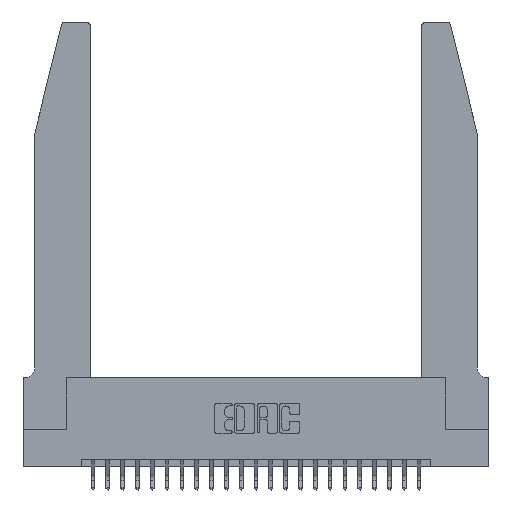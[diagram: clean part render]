
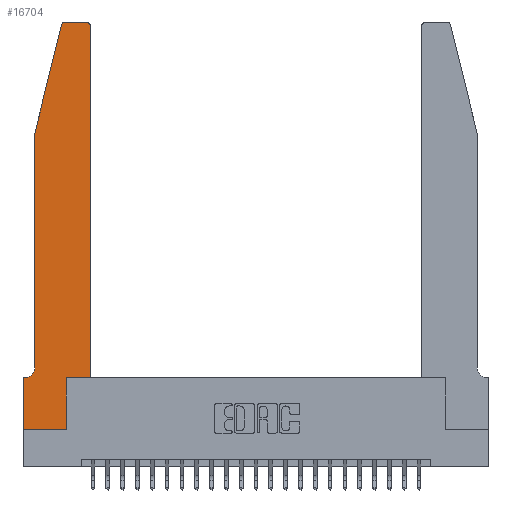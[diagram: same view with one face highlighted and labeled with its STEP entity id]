
A CAD part, top view. The second image highlights one B-rep face of the part: STEP entity #16704.
In plain terms, the highlighted planar face has unit normal (0, 0, 1).
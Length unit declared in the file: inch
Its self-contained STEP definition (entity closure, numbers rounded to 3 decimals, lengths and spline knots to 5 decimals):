
#554 = VERTEX_POINT ( 'NONE', #5459 ) ;
#1057 = EDGE_CURVE ( 'NONE', #1866, #18185, #18213, .T. ) ;
#1120 = ORIENTED_EDGE ( 'NONE', *, *, #1057, .T. ) ;
#1135 = DIRECTION ( 'NONE',  ( 0., 1., 0. ) ) ;
#1212 = DIRECTION ( 'NONE',  ( 0., 0., 1. ) ) ;
#1472 = VECTOR ( 'NONE', #25220, 39.37008 ) ;
#1668 = ORIENTED_EDGE ( 'NONE', *, *, #20051, .T. ) ;
#1866 = VERTEX_POINT ( 'NONE', #25402 ) ;
#1999 = EDGE_LOOP ( 'NONE', ( #12374, #14476, #10716, #1668, #5855, #5025, #1120, #21584, #4840, #23138, #11516, #9669 ) ) ;
#2002 = VECTOR ( 'NONE', #21650, 39.37008 ) ;
#2363 = VECTOR ( 'NONE', #12882, 39.37008 ) ;
#2982 = CARTESIAN_POINT ( 'NONE',  ( 0.4505, 0.35, 0.37 ) ) ;
#3027 = FACE_OUTER_BOUND ( 'NONE', #1999, .T. ) ;
#3102 = CARTESIAN_POINT ( 'NONE',  ( 0.2865, 0.35, 0.37 ) ) ;
#3235 = EDGE_CURVE ( 'NONE', #9959, #17209, #5210, .T. ) ;
#3626 = VECTOR ( 'NONE', #8977, 39.37008 ) ;
#4142 = VECTOR ( 'NONE', #10267, 39.37008 ) ;
#4840 = ORIENTED_EDGE ( 'NONE', *, *, #15202, .T. ) ;
#5025 = ORIENTED_EDGE ( 'NONE', *, *, #18685, .T. ) ;
#5210 = LINE ( 'NONE', #7529, #14553 ) ;
#5345 = EDGE_CURVE ( 'NONE', #22620, #9959, #12611, .T. ) ;
#5459 = CARTESIAN_POINT ( 'NONE',  ( 0.2865, 0., 0.37 ) ) ;
#5855 = ORIENTED_EDGE ( 'NONE', *, *, #17595, .T. ) ;
#5889 = CIRCLE ( 'NONE', #6001, 0.07 ) ;
#6001 = AXIS2_PLACEMENT_3D ( 'NONE', #19806, #8163, #21747 ) ;
#6195 = VECTOR ( 'NONE', #22273, 39.37008 ) ;
#6273 = CARTESIAN_POINT ( 'NONE',  ( 0.4205, 2.72, 0.37 ) ) ;
#6598 = CARTESIAN_POINT ( 'NONE',  ( 0.25487, 2.72718, 0.37 ) ) ;
#7315 = VERTEX_POINT ( 'NONE', #19235 ) ;
#7410 = VERTEX_POINT ( 'NONE', #11855 ) ;
#7475 = LINE ( 'NONE', #10089, #2002 ) ;
#7529 = CARTESIAN_POINT ( 'NONE',  ( 0.4505, 0.35, 0.37 ) ) ;
#7769 = CARTESIAN_POINT ( 'NONE',  ( 0.0755, 0.35, 0.37 ) ) ;
#8083 = CIRCLE ( 'NONE', #14499, 0.03 ) ;
#8146 = CARTESIAN_POINT ( 'NONE',  ( 0., 0., 0.37 ) ) ;
#8163 = DIRECTION ( 'NONE',  ( 0., 0., -1. ) ) ;
#8234 = CIRCLE ( 'NONE', #23222, 0.03 ) ;
#8270 = DIRECTION ( 'NONE',  ( 1., 0., 0. ) ) ;
#8977 = DIRECTION ( 'NONE',  ( 1., 0., 0. ) ) ;
#9244 = EDGE_CURVE ( 'NONE', #18185, #554, #14301, .T. ) ;
#9580 = CARTESIAN_POINT ( 'NONE',  ( 0.284, 2.72, 0.37 ) ) ;
#9669 = ORIENTED_EDGE ( 'NONE', *, *, #24172, .T. ) ;
#9959 = VERTEX_POINT ( 'NONE', #2982 ) ;
#10089 = CARTESIAN_POINT ( 'NONE',  ( 0.0755, 2., 0.37 ) ) ;
#10267 = DIRECTION ( 'NONE',  ( -0.239, -0.971, 0. ) ) ;
#10716 = ORIENTED_EDGE ( 'NONE', *, *, #11578, .T. ) ;
#11509 = LINE ( 'NONE', #16530, #6195 ) ;
#11516 = ORIENTED_EDGE ( 'NONE', *, *, #3235, .T. ) ;
#11578 = EDGE_CURVE ( 'NONE', #16018, #12915, #14186, .T. ) ;
#11592 = DIRECTION ( 'NONE',  ( 1., 0., 0. ) ) ;
#11786 = CARTESIAN_POINT ( 'NONE',  ( 0.2865, 0.35, 0.37 ) ) ;
#11855 = CARTESIAN_POINT ( 'NONE',  ( 0.0055, 0.35, 0.37 ) ) ;
#12374 = ORIENTED_EDGE ( 'NONE', *, *, #17781, .T. ) ;
#12384 = CARTESIAN_POINT ( 'NONE',  ( 0.284, 2.75, 0.37 ) ) ;
#12611 = LINE ( 'NONE', #13923, #17730 ) ;
#12840 = AXIS2_PLACEMENT_3D ( 'NONE', #20936, #1212, #15321 ) ;
#12882 = DIRECTION ( 'NONE',  ( 0., -1., 0. ) ) ;
#12915 = VERTEX_POINT ( 'NONE', #17141 ) ;
#13000 = CARTESIAN_POINT ( 'NONE',  ( 0.4505, 2.72, 0.37 ) ) ;
#13360 = PLANE ( 'NONE',  #12840 ) ;
#13923 = CARTESIAN_POINT ( 'NONE',  ( 0.4505, 0.35, 0.37 ) ) ;
#14101 = VECTOR ( 'NONE', #19444, 39.37008 ) ;
#14148 = CARTESIAN_POINT ( 'NONE',  ( 0., 0., 0.37 ) ) ;
#14186 = LINE ( 'NONE', #21837, #4142 ) ;
#14301 = LINE ( 'NONE', #16787, #3626 ) ;
#14476 = ORIENTED_EDGE ( 'NONE', *, *, #17411, .T. ) ;
#14499 = AXIS2_PLACEMENT_3D ( 'NONE', #9580, #23107, #11592 ) ;
#14553 = VECTOR ( 'NONE', #1135, 39.37008 ) ;
#15202 = EDGE_CURVE ( 'NONE', #554, #22620, #21880, .T. ) ;
#15321 = DIRECTION ( 'NONE',  ( 1., 0., 0. ) ) ;
#16018 = VERTEX_POINT ( 'NONE', #6598 ) ;
#16530 = CARTESIAN_POINT ( 'NONE',  ( 0.2605, 2.75, 0.37 ) ) ;
#16704 = ADVANCED_FACE ( 'NONE', ( #3027 ), #13360, .T. ) ;
#16787 = CARTESIAN_POINT ( 'NONE',  ( 0., 0., 0.37 ) ) ;
#17141 = CARTESIAN_POINT ( 'NONE',  ( 0.0755, 2., 0.37 ) ) ;
#17209 = VERTEX_POINT ( 'NONE', #13000 ) ;
#17411 = EDGE_CURVE ( 'NONE', #20614, #16018, #8083, .T. ) ;
#17595 = EDGE_CURVE ( 'NONE', #7315, #7410, #5889, .T. ) ;
#17730 = VECTOR ( 'NONE', #19635, 39.37008 ) ;
#17781 = EDGE_CURVE ( 'NONE', #23366, #20614, #11509, .T. ) ;
#18185 = VERTEX_POINT ( 'NONE', #8146 ) ;
#18213 = LINE ( 'NONE', #14148, #2363 ) ;
#18552 = LINE ( 'NONE', #7769, #14101 ) ;
#18685 = EDGE_CURVE ( 'NONE', #7410, #1866, #18552, .T. ) ;
#19235 = CARTESIAN_POINT ( 'NONE',  ( 0.0755, 0.42, 0.37 ) ) ;
#19444 = DIRECTION ( 'NONE',  ( -1., 0., 0. ) ) ;
#19635 = DIRECTION ( 'NONE',  ( 1., 0., 0. ) ) ;
#19806 = CARTESIAN_POINT ( 'NONE',  ( 0.0055, 0.42, 0.37 ) ) ;
#19895 = DIRECTION ( 'NONE',  ( 0., 0., 1. ) ) ;
#20051 = EDGE_CURVE ( 'NONE', #12915, #7315, #7475, .T. ) ;
#20614 = VERTEX_POINT ( 'NONE', #12384 ) ;
#20936 = CARTESIAN_POINT ( 'NONE',  ( 0., 0.35, 0.37 ) ) ;
#21584 = ORIENTED_EDGE ( 'NONE', *, *, #9244, .T. ) ;
#21650 = DIRECTION ( 'NONE',  ( 0., -1., 0. ) ) ;
#21747 = DIRECTION ( 'NONE',  ( -1., 0., 0. ) ) ;
#21837 = CARTESIAN_POINT ( 'NONE',  ( 0.0755, 2., 0.37 ) ) ;
#21880 = LINE ( 'NONE', #11786, #1472 ) ;
#22273 = DIRECTION ( 'NONE',  ( -1., 0., 0. ) ) ;
#22620 = VERTEX_POINT ( 'NONE', #3102 ) ;
#23107 = DIRECTION ( 'NONE',  ( 0., 0., 1. ) ) ;
#23138 = ORIENTED_EDGE ( 'NONE', *, *, #5345, .T. ) ;
#23222 = AXIS2_PLACEMENT_3D ( 'NONE', #6273, #19895, #8270 ) ;
#23366 = VERTEX_POINT ( 'NONE', #23395 ) ;
#23395 = CARTESIAN_POINT ( 'NONE',  ( 0.4205, 2.75, 0.37 ) ) ;
#24172 = EDGE_CURVE ( 'NONE', #17209, #23366, #8234, .T. ) ;
#25220 = DIRECTION ( 'NONE',  ( 0., 1., 0. ) ) ;
#25402 = CARTESIAN_POINT ( 'NONE',  ( 0., 0.35, 0.37 ) ) ;
